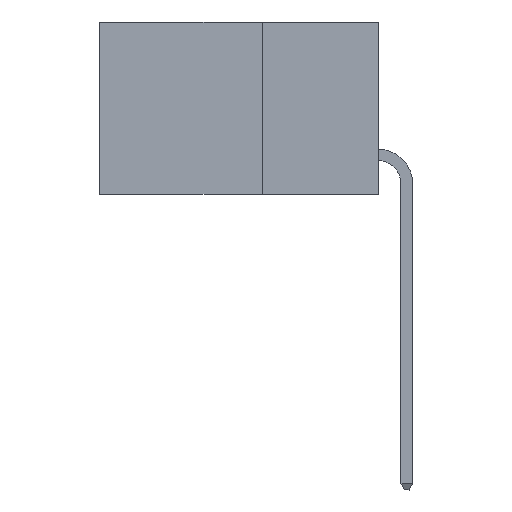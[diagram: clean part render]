
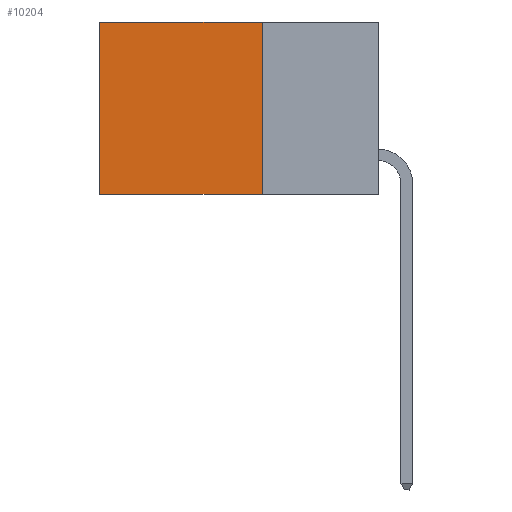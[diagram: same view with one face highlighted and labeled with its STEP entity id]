
A CAD part, left-side view. The second image highlights one B-rep face of the part: STEP entity #10204.
In plain terms, the highlighted planar face has unit normal (-1, 0, 0).
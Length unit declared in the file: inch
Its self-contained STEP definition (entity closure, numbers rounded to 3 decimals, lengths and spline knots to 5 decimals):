
#1261 = LINE ( 'NONE', #3844, #4719 ) ;
#2470 = EDGE_CURVE ( 'NONE', #2559, #10211, #7200, .T. ) ;
#2559 = VERTEX_POINT ( 'NONE', #14345 ) ;
#2727 = FACE_OUTER_BOUND ( 'NONE', #13021, .T. ) ;
#3100 = CARTESIAN_POINT ( 'NONE',  ( 0.298, 0.25, -0.37 ) ) ;
#3844 = CARTESIAN_POINT ( 'NONE',  ( 0.298, 0.6, 0. ) ) ;
#3965 = CARTESIAN_POINT ( 'NONE',  ( 0.298, 0.25, -0.37 ) ) ;
#4719 = VECTOR ( 'NONE', #10771, 39.37008 ) ;
#4813 = DIRECTION ( 'NONE',  ( 0., 0., -1. ) ) ;
#6233 = CARTESIAN_POINT ( 'NONE',  ( 0.298, 0.6, 0. ) ) ;
#7200 = LINE ( 'NONE', #10760, #12587 ) ;
#7826 = ORIENTED_EDGE ( 'NONE', *, *, #11225, .F. ) ;
#7943 = ORIENTED_EDGE ( 'NONE', *, *, #2470, .T. ) ;
#8121 = LINE ( 'NONE', #3100, #11990 ) ;
#9137 = PLANE ( 'NONE',  #16439 ) ;
#9199 = CARTESIAN_POINT ( 'NONE',  ( 0.298, 0.25, 0. ) ) ;
#9865 = ORIENTED_EDGE ( 'NONE', *, *, #10803, .F. ) ;
#10204 = ADVANCED_FACE ( 'NONE', ( #2727 ), #9137, .F. ) ;
#10211 = VERTEX_POINT ( 'NONE', #6233 ) ;
#10444 = CARTESIAN_POINT ( 'NONE',  ( 0.298, 0.25, 0. ) ) ;
#10760 = CARTESIAN_POINT ( 'NONE',  ( 0.298, 0.25, 0. ) ) ;
#10771 = DIRECTION ( 'NONE',  ( 0., 0., -1. ) ) ;
#10803 = EDGE_CURVE ( 'NONE', #12344, #14153, #8121, .T. ) ;
#11225 = EDGE_CURVE ( 'NONE', #2559, #12344, #14334, .T. ) ;
#11878 = DIRECTION ( 'NONE',  ( 1., 0., 0. ) ) ;
#11990 = VECTOR ( 'NONE', #12768, 39.37008 ) ;
#12344 = VERTEX_POINT ( 'NONE', #3965 ) ;
#12587 = VECTOR ( 'NONE', #17047, 39.37008 ) ;
#12768 = DIRECTION ( 'NONE',  ( 0., 1., 0. ) ) ;
#13021 = EDGE_LOOP ( 'NONE', ( #15765, #9865, #7826, #7943 ) ) ;
#13253 = DIRECTION ( 'NONE',  ( 0., 0., -1. ) ) ;
#14153 = VERTEX_POINT ( 'NONE', #17512 ) ;
#14334 = LINE ( 'NONE', #9199, #16498 ) ;
#14345 = CARTESIAN_POINT ( 'NONE',  ( 0.298, 0.25, 0. ) ) ;
#14573 = EDGE_CURVE ( 'NONE', #10211, #14153, #1261, .T. ) ;
#15765 = ORIENTED_EDGE ( 'NONE', *, *, #14573, .T. ) ;
#16439 = AXIS2_PLACEMENT_3D ( 'NONE', #10444, #11878, #4813 ) ;
#16498 = VECTOR ( 'NONE', #13253, 39.37008 ) ;
#17047 = DIRECTION ( 'NONE',  ( 0., 1., 0. ) ) ;
#17512 = CARTESIAN_POINT ( 'NONE',  ( 0.298, 0.6, -0.37 ) ) ;
